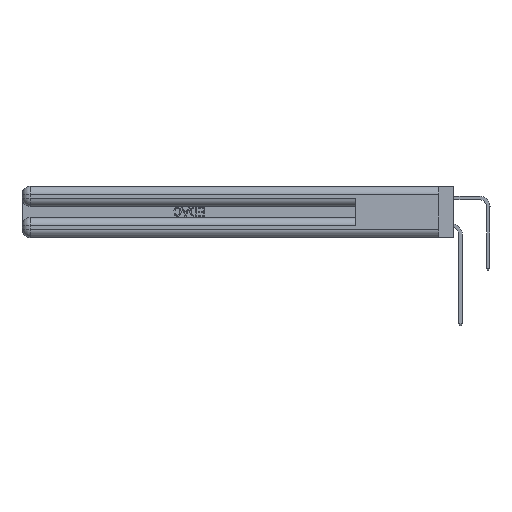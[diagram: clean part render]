
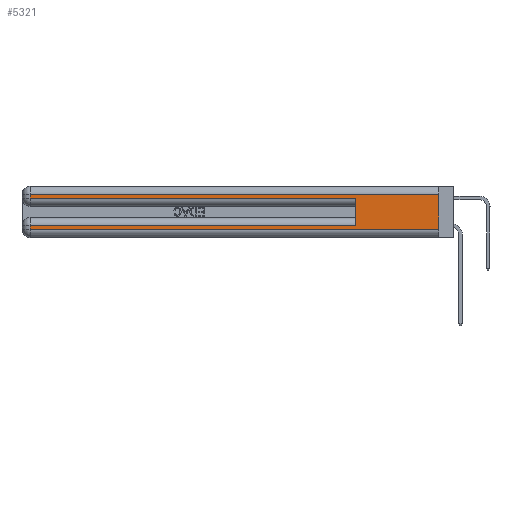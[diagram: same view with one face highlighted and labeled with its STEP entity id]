
A CAD part, left-side view. The second image highlights one B-rep face of the part: STEP entity #5321.
In plain terms, the highlighted planar face has unit normal (-1, 0, 0).
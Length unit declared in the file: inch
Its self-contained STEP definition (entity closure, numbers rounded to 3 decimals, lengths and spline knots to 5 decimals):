
#329 = LINE ( 'NONE', #28758, #21212 ) ;
#1329 = VERTEX_POINT ( 'NONE', #26456 ) ;
#2333 = DIRECTION ( 'NONE',  ( 0., -1., 0. ) ) ;
#2399 = ORIENTED_EDGE ( 'NONE', *, *, #42190, .T. ) ;
#2709 = CARTESIAN_POINT ( 'NONE',  ( 0., 2.94, 0.06 ) ) ;
#4513 = VECTOR ( 'NONE', #25965, 39.37008 ) ;
#4744 = DIRECTION ( 'NONE',  ( 0., 0., -1. ) ) ;
#4891 = PLANE ( 'NONE',  #9359 ) ;
#5193 = VERTEX_POINT ( 'NONE', #24005 ) ;
#5321 = ADVANCED_FACE ( 'NONE', ( #36163 ), #4891, .F. ) ;
#5771 = LINE ( 'NONE', #33818, #40250 ) ;
#5864 = ORIENTED_EDGE ( 'NONE', *, *, #24308, .T. ) ;
#7482 = CARTESIAN_POINT ( 'NONE',  ( 0., 0., 0.37 ) ) ;
#8144 = CARTESIAN_POINT ( 'NONE',  ( 0., 2.94, 0.285 ) ) ;
#8259 = EDGE_CURVE ( 'NONE', #1329, #16310, #34159, .T. ) ;
#9359 = AXIS2_PLACEMENT_3D ( 'NONE', #31075, #34591, #4744 ) ;
#10547 = DIRECTION ( 'NONE',  ( 0., 0., -1. ) ) ;
#11081 = ORIENTED_EDGE ( 'NONE', *, *, #34098, .T. ) ;
#11492 = EDGE_CURVE ( 'NONE', #43124, #31429, #35490, .T. ) ;
#11649 = LINE ( 'NONE', #33082, #29963 ) ;
#12509 = CARTESIAN_POINT ( 'NONE',  ( 0., 0., 0.285 ) ) ;
#15458 = CARTESIAN_POINT ( 'NONE',  ( 0., 0.6, 0.145 ) ) ;
#15703 = DIRECTION ( 'NONE',  ( 0., 1., 0. ) ) ;
#16310 = VERTEX_POINT ( 'NONE', #26910 ) ;
#17094 = CARTESIAN_POINT ( 'NONE',  ( 0., 0., 0.085 ) ) ;
#18904 = CARTESIAN_POINT ( 'NONE',  ( 0., 0., 0.31 ) ) ;
#18954 = ORIENTED_EDGE ( 'NONE', *, *, #29955, .T. ) ;
#21212 = VECTOR ( 'NONE', #2333, 39.37008 ) ;
#21610 = VERTEX_POINT ( 'NONE', #2709 ) ;
#21732 = CARTESIAN_POINT ( 'NONE',  ( 0., 2.94, 0.085 ) ) ;
#22248 = CARTESIAN_POINT ( 'NONE',  ( 0., 0., 0.31 ) ) ;
#22698 = EDGE_CURVE ( 'NONE', #28937, #16310, #31190, .T. ) ;
#24005 = CARTESIAN_POINT ( 'NONE',  ( 0., 2.94, 0.31 ) ) ;
#24167 = VECTOR ( 'NONE', #35608, 39.37008 ) ;
#24235 = ORIENTED_EDGE ( 'NONE', *, *, #11492, .F. ) ;
#24308 = EDGE_CURVE ( 'NONE', #43124, #5193, #29934, .T. ) ;
#25496 = VECTOR ( 'NONE', #27068, 39.37008 ) ;
#25965 = DIRECTION ( 'NONE',  ( 0., -1., 0. ) ) ;
#26456 = CARTESIAN_POINT ( 'NONE',  ( 0., 0.6, 0.085 ) ) ;
#26816 = VECTOR ( 'NONE', #15703, 39.37008 ) ;
#26910 = CARTESIAN_POINT ( 'NONE',  ( 0., 0.6, 0.285 ) ) ;
#27068 = DIRECTION ( 'NONE',  ( 0., 0., -1. ) ) ;
#28758 = CARTESIAN_POINT ( 'NONE',  ( 0., 0., 0.06 ) ) ;
#28937 = VERTEX_POINT ( 'NONE', #8144 ) ;
#29701 = CARTESIAN_POINT ( 'NONE',  ( 0., 0., 0.06 ) ) ;
#29934 = LINE ( 'NONE', #22248, #24167 ) ;
#29955 = EDGE_CURVE ( 'NONE', #21610, #31429, #329, .T. ) ;
#29963 = VECTOR ( 'NONE', #10547, 39.37008 ) ;
#31075 = CARTESIAN_POINT ( 'NONE',  ( 0., 0., 0.37 ) ) ;
#31190 = LINE ( 'NONE', #12509, #4513 ) ;
#31429 = VERTEX_POINT ( 'NONE', #29701 ) ;
#32642 = EDGE_CURVE ( 'NONE', #1329, #34473, #35733, .T. ) ;
#32786 = DIRECTION ( 'NONE',  ( 0., 0., -1. ) ) ;
#33082 = CARTESIAN_POINT ( 'NONE',  ( 0., 2.94, 0.37 ) ) ;
#33155 = EDGE_LOOP ( 'NONE', ( #24235, #5864, #2399, #40934, #42387, #42515, #11081, #18954 ) ) ;
#33818 = CARTESIAN_POINT ( 'NONE',  ( 0., 2.94, 0.37 ) ) ;
#34098 = EDGE_CURVE ( 'NONE', #34473, #21610, #5771, .T. ) ;
#34159 = LINE ( 'NONE', #15458, #41168 ) ;
#34473 = VERTEX_POINT ( 'NONE', #21732 ) ;
#34591 = DIRECTION ( 'NONE',  ( 1., 0., 0. ) ) ;
#35490 = LINE ( 'NONE', #7482, #25496 ) ;
#35608 = DIRECTION ( 'NONE',  ( 0., 1., 0. ) ) ;
#35733 = LINE ( 'NONE', #17094, #26816 ) ;
#36163 = FACE_OUTER_BOUND ( 'NONE', #33155, .T. ) ;
#40250 = VECTOR ( 'NONE', #32786, 39.37008 ) ;
#40934 = ORIENTED_EDGE ( 'NONE', *, *, #22698, .T. ) ;
#41168 = VECTOR ( 'NONE', #42486, 39.37008 ) ;
#42190 = EDGE_CURVE ( 'NONE', #5193, #28937, #11649, .T. ) ;
#42387 = ORIENTED_EDGE ( 'NONE', *, *, #8259, .F. ) ;
#42486 = DIRECTION ( 'NONE',  ( 0., 0., 1. ) ) ;
#42515 = ORIENTED_EDGE ( 'NONE', *, *, #32642, .T. ) ;
#43124 = VERTEX_POINT ( 'NONE', #18904 ) ;
